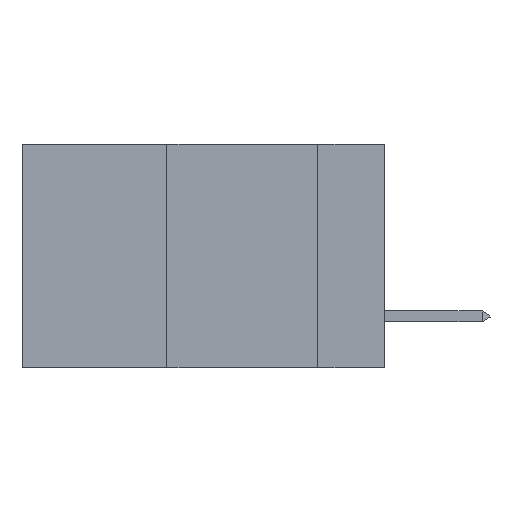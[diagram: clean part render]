
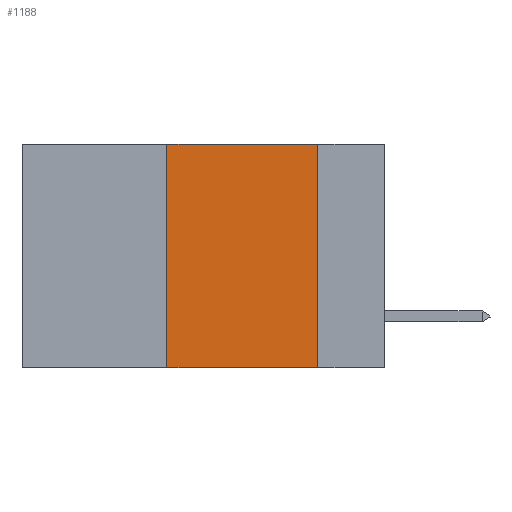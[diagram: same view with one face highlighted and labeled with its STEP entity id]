
A CAD part, left-side view. The second image highlights one B-rep face of the part: STEP entity #1188.
In plain terms, the highlighted planar face has unit normal (-1, 0, 0).
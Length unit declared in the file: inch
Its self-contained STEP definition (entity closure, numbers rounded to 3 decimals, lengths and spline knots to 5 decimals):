
#1188 = ADVANCED_FACE ( 'NONE', ( #24239 ), #25875, .F. ) ;
#2017 = CARTESIAN_POINT ( 'NONE',  ( 0., 0.11, -0.37 ) ) ;
#3925 = ORIENTED_EDGE ( 'NONE', *, *, #45811, .F. ) ;
#5273 = CARTESIAN_POINT ( 'NONE',  ( 0., 0.6, -0.37 ) ) ;
#9292 = VERTEX_POINT ( 'NONE', #13050 ) ;
#11028 = CARTESIAN_POINT ( 'NONE',  ( 0., 0.11, 0. ) ) ;
#11181 = DIRECTION ( 'NONE',  ( 0., 0., -1. ) ) ;
#11560 = LINE ( 'NONE', #5273, #28448 ) ;
#12051 = AXIS2_PLACEMENT_3D ( 'NONE', #29821, #40514, #44093 ) ;
#12138 = EDGE_LOOP ( 'NONE', ( #32361, #3925, #22451, #45055 ) ) ;
#13050 = CARTESIAN_POINT ( 'NONE',  ( 0., 0.36, -0.37 ) ) ;
#14500 = LINE ( 'NONE', #43737, #22358 ) ;
#18122 = VECTOR ( 'NONE', #11181, 39.37008 ) ;
#20374 = VERTEX_POINT ( 'NONE', #2017 ) ;
#20740 = CARTESIAN_POINT ( 'NONE',  ( 0., 0.36, 0. ) ) ;
#22358 = VECTOR ( 'NONE', #40126, 39.37008 ) ;
#22451 = ORIENTED_EDGE ( 'NONE', *, *, #43633, .F. ) ;
#23228 = DIRECTION ( 'NONE',  ( 0., -1., 0. ) ) ;
#24239 = FACE_OUTER_BOUND ( 'NONE', #12138, .T. ) ;
#25875 = PLANE ( 'NONE',  #12051 ) ;
#27620 = LINE ( 'NONE', #20740, #36663 ) ;
#28448 = VECTOR ( 'NONE', #23228, 39.37008 ) ;
#29281 = CARTESIAN_POINT ( 'NONE',  ( 0., 0.36, 0. ) ) ;
#29670 = EDGE_CURVE ( 'NONE', #42369, #20374, #44005, .T. ) ;
#29821 = CARTESIAN_POINT ( 'NONE',  ( 0., 0.6, 0. ) ) ;
#32361 = ORIENTED_EDGE ( 'NONE', *, *, #29670, .F. ) ;
#34276 = CARTESIAN_POINT ( 'NONE',  ( 0., 0.11, 0. ) ) ;
#36663 = VECTOR ( 'NONE', #45610, 39.37008 ) ;
#40126 = DIRECTION ( 'NONE',  ( 0., -1., 0. ) ) ;
#40514 = DIRECTION ( 'NONE',  ( 1., 0., 0. ) ) ;
#42369 = VERTEX_POINT ( 'NONE', #34276 ) ;
#43633 = EDGE_CURVE ( 'NONE', #9292, #45927, #27620, .T. ) ;
#43737 = CARTESIAN_POINT ( 'NONE',  ( 0., 0.6, 0. ) ) ;
#44005 = LINE ( 'NONE', #11028, #18122 ) ;
#44093 = DIRECTION ( 'NONE',  ( 0., 0., -1. ) ) ;
#45055 = ORIENTED_EDGE ( 'NONE', *, *, #46688, .T. ) ;
#45610 = DIRECTION ( 'NONE',  ( 0., 0., 1. ) ) ;
#45811 = EDGE_CURVE ( 'NONE', #45927, #42369, #14500, .T. ) ;
#45927 = VERTEX_POINT ( 'NONE', #29281 ) ;
#46688 = EDGE_CURVE ( 'NONE', #9292, #20374, #11560, .T. ) ;
